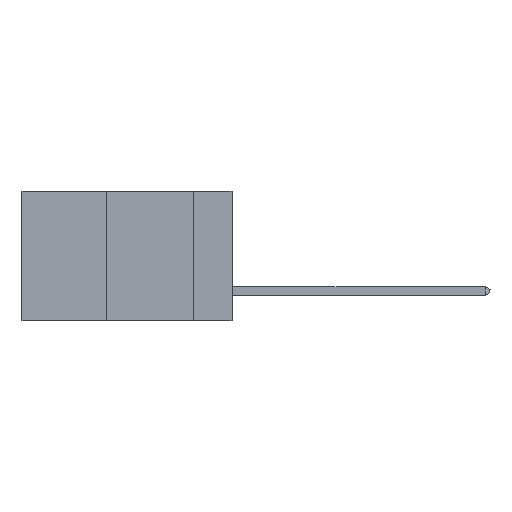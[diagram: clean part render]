
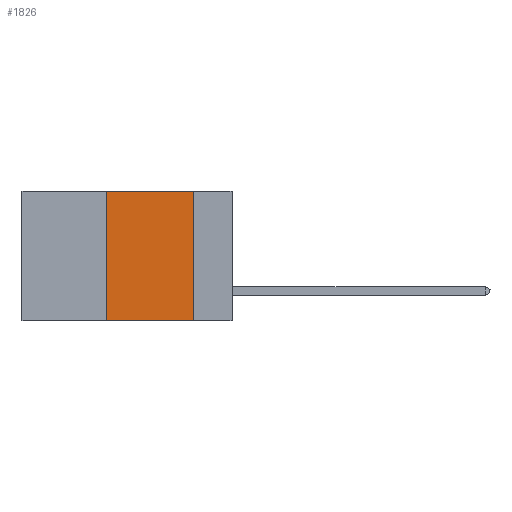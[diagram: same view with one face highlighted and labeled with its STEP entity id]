
A CAD part, left-side view. The second image highlights one B-rep face of the part: STEP entity #1826.
In plain terms, the highlighted planar face has unit normal (-1, 0, 0).
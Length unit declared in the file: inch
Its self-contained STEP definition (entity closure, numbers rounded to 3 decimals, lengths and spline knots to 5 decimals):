
#701 = CARTESIAN_POINT ( 'NONE',  ( 0., 0.36, 0. ) ) ;
#1826 = ADVANCED_FACE ( 'NONE', ( #29745 ), #4684, .F. ) ;
#2448 = CARTESIAN_POINT ( 'NONE',  ( 0., 0.36, 0. ) ) ;
#2599 = ORIENTED_EDGE ( 'NONE', *, *, #40532, .F. ) ;
#2988 = LINE ( 'NONE', #37140, #43059 ) ;
#3952 = DIRECTION ( 'NONE',  ( 0., -1., 0. ) ) ;
#4684 = PLANE ( 'NONE',  #19558 ) ;
#4701 = ORIENTED_EDGE ( 'NONE', *, *, #17590, .T. ) ;
#5702 = ORIENTED_EDGE ( 'NONE', *, *, #43176, .F. ) ;
#6436 = ORIENTED_EDGE ( 'NONE', *, *, #7901, .F. ) ;
#7901 = EDGE_CURVE ( 'NONE', #31283, #17988, #32019, .T. ) ;
#9154 = VERTEX_POINT ( 'NONE', #44118 ) ;
#11590 = LINE ( 'NONE', #23178, #48138 ) ;
#15880 = DIRECTION ( 'NONE',  ( 1., 0., 0. ) ) ;
#16203 = DIRECTION ( 'NONE',  ( 0., 0., -1. ) ) ;
#17258 = VECTOR ( 'NONE', #42513, 39.37008 ) ;
#17398 = CARTESIAN_POINT ( 'NONE',  ( 0., 0.11, 0. ) ) ;
#17590 = EDGE_CURVE ( 'NONE', #31283, #9154, #24533, .T. ) ;
#17988 = VERTEX_POINT ( 'NONE', #2448 ) ;
#18633 = DIRECTION ( 'NONE',  ( 0., 0., -1. ) ) ;
#19558 = AXIS2_PLACEMENT_3D ( 'NONE', #31559, #15880, #16203 ) ;
#22910 = CARTESIAN_POINT ( 'NONE',  ( 0., 0.36, -0.37 ) ) ;
#23178 = CARTESIAN_POINT ( 'NONE',  ( 0., 0.6, 0. ) ) ;
#24533 = LINE ( 'NONE', #30334, #45198 ) ;
#29745 = FACE_OUTER_BOUND ( 'NONE', #31729, .T. ) ;
#30334 = CARTESIAN_POINT ( 'NONE',  ( 0., 0.6, -0.37 ) ) ;
#31283 = VERTEX_POINT ( 'NONE', #22910 ) ;
#31559 = CARTESIAN_POINT ( 'NONE',  ( 0., 0.6, 0. ) ) ;
#31729 = EDGE_LOOP ( 'NONE', ( #5702, #2599, #6436, #4701 ) ) ;
#32019 = LINE ( 'NONE', #701, #17258 ) ;
#37140 = CARTESIAN_POINT ( 'NONE',  ( 0., 0.11, 0. ) ) ;
#40532 = EDGE_CURVE ( 'NONE', #17988, #45413, #11590, .T. ) ;
#41992 = DIRECTION ( 'NONE',  ( 0., -1., 0. ) ) ;
#42513 = DIRECTION ( 'NONE',  ( 0., 0., 1. ) ) ;
#43059 = VECTOR ( 'NONE', #18633, 39.37008 ) ;
#43176 = EDGE_CURVE ( 'NONE', #45413, #9154, #2988, .T. ) ;
#44118 = CARTESIAN_POINT ( 'NONE',  ( 0., 0.11, -0.37 ) ) ;
#45198 = VECTOR ( 'NONE', #41992, 39.37008 ) ;
#45413 = VERTEX_POINT ( 'NONE', #17398 ) ;
#48138 = VECTOR ( 'NONE', #3952, 39.37008 ) ;
